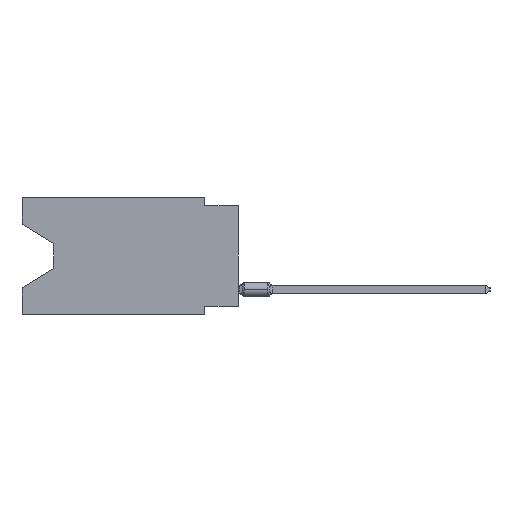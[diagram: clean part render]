
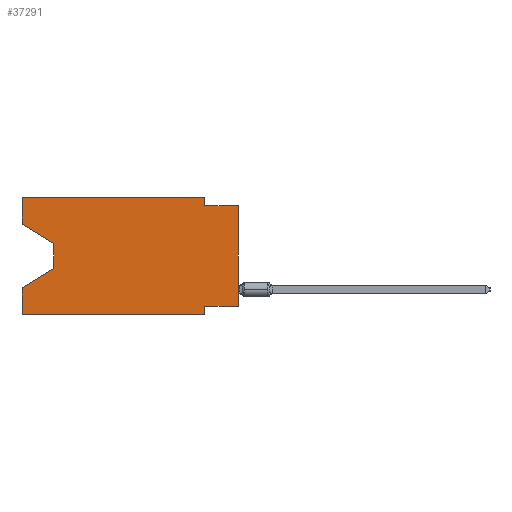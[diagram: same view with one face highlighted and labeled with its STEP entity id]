
A CAD part, left-side view. The second image highlights one B-rep face of the part: STEP entity #37291.
In plain terms, the highlighted planar face has unit normal (-1, 0, 0).
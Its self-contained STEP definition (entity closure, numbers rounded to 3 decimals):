
#938 = VERTEX_POINT ( 'NONE', #22736 ) ;
#1306 = VERTEX_POINT ( 'NONE', #23757 ) ;
#2933 = DIRECTION ( 'NONE',  ( 0., -0.855, -0.519 ) ) ;
#4351 = DIRECTION ( 'NONE',  ( 0., 0., -1. ) ) ;
#4846 = EDGE_CURVE ( 'NONE', #21791, #79391, #37138, .T. ) ;
#6887 = VECTOR ( 'NONE', #43205, 1000. ) ;
#7456 = CARTESIAN_POINT ( 'NONE',  ( 0., 13.97, -5.385 ) ) ;
#8597 = DIRECTION ( 'NONE',  ( 0., 1., 0. ) ) ;
#9019 = VERTEX_POINT ( 'NONE', #7456 ) ;
#9410 = CARTESIAN_POINT ( 'NONE',  ( 0., 0., -8.255 ) ) ;
#10140 = EDGE_CURVE ( 'NONE', #9019, #41474, #44554, .T. ) ;
#10572 = VERTEX_POINT ( 'NONE', #30874 ) ;
#11538 = EDGE_CURVE ( 'NONE', #79391, #1306, #14643, .T. ) ;
#13422 = VECTOR ( 'NONE', #35236, 1000. ) ;
#14043 = CARTESIAN_POINT ( 'NONE',  ( 0., 2.54, 0. ) ) ;
#14643 = LINE ( 'NONE', #39780, #13422 ) ;
#15693 = VECTOR ( 'NONE', #2933, 1000. ) ;
#16587 = CARTESIAN_POINT ( 'NONE',  ( 0., 16.383, -6.852 ) ) ;
#17521 = CARTESIAN_POINT ( 'NONE',  ( 0., 0., -8.255 ) ) ;
#18302 = DIRECTION ( 'NONE',  ( 0., 0., -1. ) ) ;
#18307 = EDGE_CURVE ( 'NONE', #57778, #63360, #47327, .T. ) ;
#21729 = VERTEX_POINT ( 'NONE', #38349 ) ;
#21738 = ORIENTED_EDGE ( 'NONE', *, *, #34671, .F. ) ;
#21791 = VERTEX_POINT ( 'NONE', #14043 ) ;
#22736 = CARTESIAN_POINT ( 'NONE',  ( 0., 16.383, -2.038 ) ) ;
#23185 = VECTOR ( 'NONE', #23950, 1000. ) ;
#23757 = CARTESIAN_POINT ( 'NONE',  ( 0., 0., -0.635 ) ) ;
#23950 = DIRECTION ( 'NONE',  ( 0., 0., -1. ) ) ;
#24711 = CARTESIAN_POINT ( 'NONE',  ( 0., 2.54, -8.89 ) ) ;
#25326 = VERTEX_POINT ( 'NONE', #64346 ) ;
#25683 = VERTEX_POINT ( 'NONE', #24711 ) ;
#26002 = FACE_OUTER_BOUND ( 'NONE', #54532, .T. ) ;
#27000 = LINE ( 'NONE', #65339, #78260 ) ;
#27525 = VECTOR ( 'NONE', #18302, 1000. ) ;
#30874 = CARTESIAN_POINT ( 'NONE',  ( 0., 16.383, -8.89 ) ) ;
#31364 = CARTESIAN_POINT ( 'NONE',  ( 0., 2.54, 0. ) ) ;
#33123 = LINE ( 'NONE', #38104, #58473 ) ;
#34641 = AXIS2_PLACEMENT_3D ( 'NONE', #37552, #44542, #68474 ) ;
#34671 = EDGE_CURVE ( 'NONE', #25326, #21791, #61760, .T. ) ;
#35236 = DIRECTION ( 'NONE',  ( 0., -1., 0. ) ) ;
#35622 = ORIENTED_EDGE ( 'NONE', *, *, #4846, .F. ) ;
#35656 = LINE ( 'NONE', #60795, #37576 ) ;
#36100 = VECTOR ( 'NONE', #8597, 1000. ) ;
#36634 = EDGE_CURVE ( 'NONE', #938, #25326, #27000, .T. ) ;
#37138 = LINE ( 'NONE', #31364, #23185 ) ;
#37291 = ADVANCED_FACE ( 'NONE', ( #26002 ), #68872, .F. ) ;
#37552 = CARTESIAN_POINT ( 'NONE',  ( 0., 16.383, 0. ) ) ;
#37576 = VECTOR ( 'NONE', #4351, 1000. ) ;
#38104 = CARTESIAN_POINT ( 'NONE',  ( 0., 16.383, -8.89 ) ) ;
#38349 = CARTESIAN_POINT ( 'NONE',  ( 0., 13.97, -3.505 ) ) ;
#39780 = CARTESIAN_POINT ( 'NONE',  ( 0., 0., -0.635 ) ) ;
#41474 = VERTEX_POINT ( 'NONE', #16587 ) ;
#43038 = LINE ( 'NONE', #54181, #27525 ) ;
#43205 = DIRECTION ( 'NONE',  ( 0., -1., 0. ) ) ;
#44542 = DIRECTION ( 'NONE',  ( 1., 0., 0. ) ) ;
#44554 = LINE ( 'NONE', #75898, #66103 ) ;
#46202 = LINE ( 'NONE', #71336, #61810 ) ;
#47327 = LINE ( 'NONE', #9410, #36100 ) ;
#48865 = DIRECTION ( 'NONE',  ( 0., 0., 1. ) ) ;
#49028 = ORIENTED_EDGE ( 'NONE', *, *, #58844, .T. ) ;
#49676 = ORIENTED_EDGE ( 'NONE', *, *, #71807, .T. ) ;
#51297 = DIRECTION ( 'NONE',  ( 0., -1., 0. ) ) ;
#52647 = EDGE_CURVE ( 'NONE', #10572, #41474, #61648, .T. ) ;
#52784 = LINE ( 'NONE', #70519, #15693 ) ;
#53174 = VECTOR ( 'NONE', #48865, 1000. ) ;
#53256 = ORIENTED_EDGE ( 'NONE', *, *, #18307, .F. ) ;
#54181 = CARTESIAN_POINT ( 'NONE',  ( 0., 13.97, -3.505 ) ) ;
#54532 = EDGE_LOOP ( 'NONE', ( #73632, #62017, #71353, #58860, #49028, #66928, #53256, #49676, #78295, #35622, #21738, #59647 ) ) ;
#57778 = VERTEX_POINT ( 'NONE', #17521 ) ;
#58129 = DIRECTION ( 'NONE',  ( 0., 0.855, -0.519 ) ) ;
#58473 = VECTOR ( 'NONE', #51297, 1000. ) ;
#58844 = EDGE_CURVE ( 'NONE', #10572, #25683, #33123, .T. ) ;
#58860 = ORIENTED_EDGE ( 'NONE', *, *, #52647, .F. ) ;
#59647 = ORIENTED_EDGE ( 'NONE', *, *, #36634, .F. ) ;
#60537 = CARTESIAN_POINT ( 'NONE',  ( 0., 16.383, 0. ) ) ;
#60795 = CARTESIAN_POINT ( 'NONE',  ( 0., 2.54, -8.89 ) ) ;
#61648 = LINE ( 'NONE', #63988, #53174 ) ;
#61760 = LINE ( 'NONE', #60537, #6887 ) ;
#61810 = VECTOR ( 'NONE', #63935, 1000. ) ;
#62017 = ORIENTED_EDGE ( 'NONE', *, *, #77485, .T. ) ;
#63360 = VERTEX_POINT ( 'NONE', #80884 ) ;
#63935 = DIRECTION ( 'NONE',  ( 0., 0., 1. ) ) ;
#63988 = CARTESIAN_POINT ( 'NONE',  ( 0., 16.383, 0. ) ) ;
#64346 = CARTESIAN_POINT ( 'NONE',  ( 0., 16.383, 0. ) ) ;
#65339 = CARTESIAN_POINT ( 'NONE',  ( 0., 16.383, 0. ) ) ;
#66103 = VECTOR ( 'NONE', #58129, 1000. ) ;
#66928 = ORIENTED_EDGE ( 'NONE', *, *, #67321, .F. ) ;
#67321 = EDGE_CURVE ( 'NONE', #63360, #25683, #35656, .T. ) ;
#67541 = CARTESIAN_POINT ( 'NONE',  ( 0., 2.54, -0.635 ) ) ;
#68474 = DIRECTION ( 'NONE',  ( 0., 0., -1. ) ) ;
#68872 = PLANE ( 'NONE',  #34641 ) ;
#70519 = CARTESIAN_POINT ( 'NONE',  ( 0., 16.383, -2.038 ) ) ;
#71336 = CARTESIAN_POINT ( 'NONE',  ( 0., 0., 0. ) ) ;
#71353 = ORIENTED_EDGE ( 'NONE', *, *, #10140, .T. ) ;
#71807 = EDGE_CURVE ( 'NONE', #57778, #1306, #46202, .T. ) ;
#73632 = ORIENTED_EDGE ( 'NONE', *, *, #78237, .T. ) ;
#75898 = CARTESIAN_POINT ( 'NONE',  ( 0., 13.97, -5.385 ) ) ;
#77485 = EDGE_CURVE ( 'NONE', #21729, #9019, #43038, .T. ) ;
#78102 = DIRECTION ( 'NONE',  ( 0., 0., 1. ) ) ;
#78237 = EDGE_CURVE ( 'NONE', #938, #21729, #52784, .T. ) ;
#78260 = VECTOR ( 'NONE', #78102, 1000. ) ;
#78295 = ORIENTED_EDGE ( 'NONE', *, *, #11538, .F. ) ;
#79391 = VERTEX_POINT ( 'NONE', #67541 ) ;
#80884 = CARTESIAN_POINT ( 'NONE',  ( 0., 2.54, -8.255 ) ) ;
